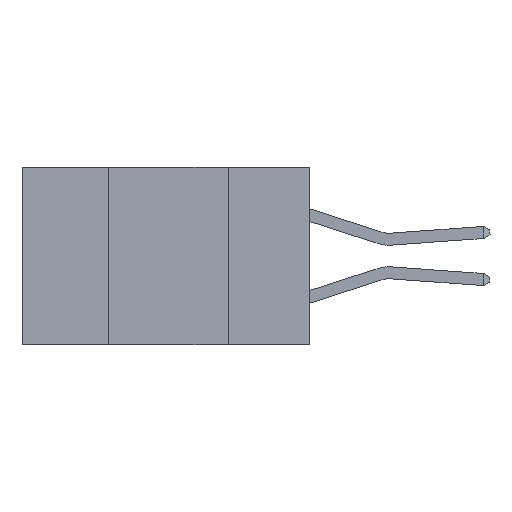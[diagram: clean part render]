
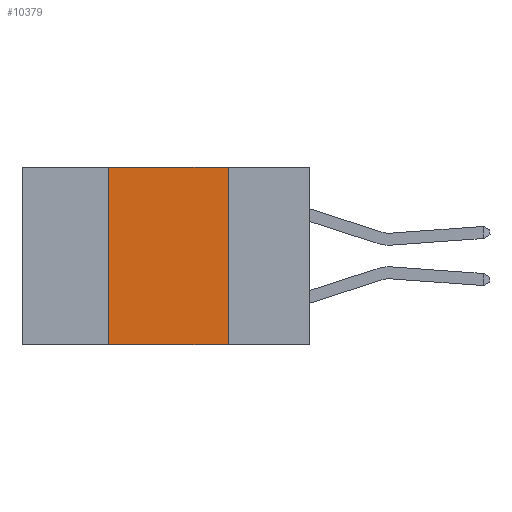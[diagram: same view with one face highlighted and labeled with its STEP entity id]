
A CAD part, left-side view. The second image highlights one B-rep face of the part: STEP entity #10379.
In plain terms, the highlighted planar face has unit normal (-1, 0, 0).
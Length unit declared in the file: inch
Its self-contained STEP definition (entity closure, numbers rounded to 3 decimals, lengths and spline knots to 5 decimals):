
#493 = DIRECTION ( 'NONE',  ( 0., -1., 0. ) ) ;
#1037 = VERTEX_POINT ( 'NONE', #6721 ) ;
#1302 = VECTOR ( 'NONE', #7835, 39.37008 ) ;
#1942 = EDGE_CURVE ( 'NONE', #5796, #5323, #11851, .T. ) ;
#3073 = ORIENTED_EDGE ( 'NONE', *, *, #6393, .F. ) ;
#3637 = EDGE_CURVE ( 'NONE', #7157, #1037, #11237, .T. ) ;
#3656 = LINE ( 'NONE', #6819, #10930 ) ;
#3734 = VECTOR ( 'NONE', #493, 39.37008 ) ;
#3792 = LINE ( 'NONE', #7664, #1302 ) ;
#3859 = CARTESIAN_POINT ( 'NONE',  ( 0., 0.42, -0.37 ) ) ;
#4168 = AXIS2_PLACEMENT_3D ( 'NONE', #4226, #5164, #11780 ) ;
#4226 = CARTESIAN_POINT ( 'NONE',  ( 0., 0.6, 0. ) ) ;
#4987 = DIRECTION ( 'NONE',  ( 0., -1., 0. ) ) ;
#5164 = DIRECTION ( 'NONE',  ( 1., 0., 0. ) ) ;
#5323 = VERTEX_POINT ( 'NONE', #7566 ) ;
#5342 = FACE_OUTER_BOUND ( 'NONE', #7316, .T. ) ;
#5557 = ORIENTED_EDGE ( 'NONE', *, *, #1942, .F. ) ;
#5750 = EDGE_CURVE ( 'NONE', #7157, #5796, #3656, .T. ) ;
#5796 = VERTEX_POINT ( 'NONE', #6441 ) ;
#5855 = ORIENTED_EDGE ( 'NONE', *, *, #5750, .F. ) ;
#6153 = ORIENTED_EDGE ( 'NONE', *, *, #3637, .T. ) ;
#6393 = EDGE_CURVE ( 'NONE', #5323, #1037, #3792, .T. ) ;
#6441 = CARTESIAN_POINT ( 'NONE',  ( 0., 0.42, 0. ) ) ;
#6583 = CARTESIAN_POINT ( 'NONE',  ( 0., 0.6, -0.37 ) ) ;
#6721 = CARTESIAN_POINT ( 'NONE',  ( 0., 0.17, -0.37 ) ) ;
#6819 = CARTESIAN_POINT ( 'NONE',  ( 0., 0.42, 0. ) ) ;
#7065 = CARTESIAN_POINT ( 'NONE',  ( 0., 0.6, 0. ) ) ;
#7157 = VERTEX_POINT ( 'NONE', #3859 ) ;
#7316 = EDGE_LOOP ( 'NONE', ( #3073, #5557, #5855, #6153 ) ) ;
#7566 = CARTESIAN_POINT ( 'NONE',  ( 0., 0.17, 0. ) ) ;
#7664 = CARTESIAN_POINT ( 'NONE',  ( 0., 0.17, 0. ) ) ;
#7818 = DIRECTION ( 'NONE',  ( 0., 0., 1. ) ) ;
#7835 = DIRECTION ( 'NONE',  ( 0., 0., -1. ) ) ;
#9939 = PLANE ( 'NONE',  #4168 ) ;
#10379 = ADVANCED_FACE ( 'NONE', ( #5342 ), #9939, .F. ) ;
#10930 = VECTOR ( 'NONE', #7818, 39.37008 ) ;
#10960 = VECTOR ( 'NONE', #4987, 39.37008 ) ;
#11237 = LINE ( 'NONE', #6583, #10960 ) ;
#11780 = DIRECTION ( 'NONE',  ( 0., 0., -1. ) ) ;
#11851 = LINE ( 'NONE', #7065, #3734 ) ;
